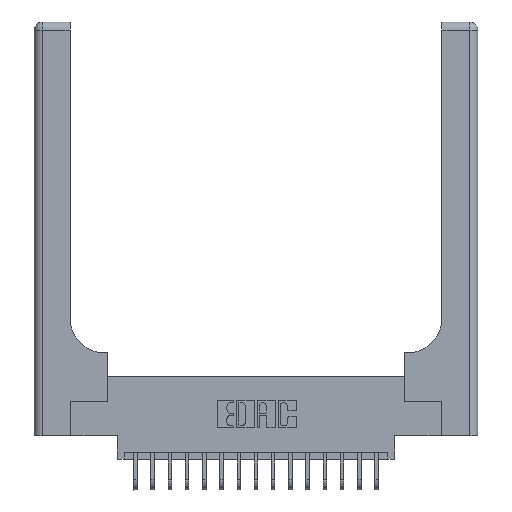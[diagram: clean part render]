
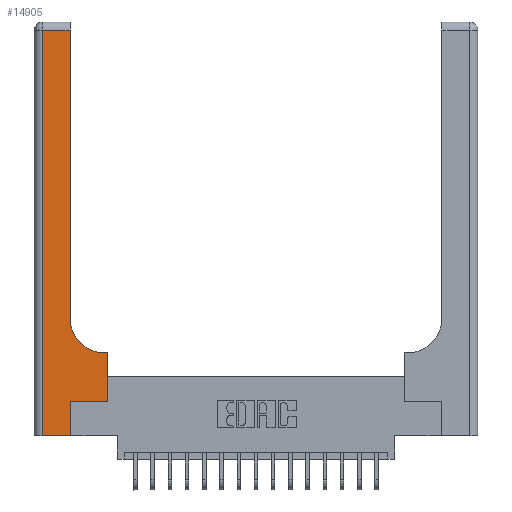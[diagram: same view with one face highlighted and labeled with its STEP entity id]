
A CAD part, top view. The second image highlights one B-rep face of the part: STEP entity #14905.
In plain terms, the highlighted planar face has unit normal (0, 0, 1).
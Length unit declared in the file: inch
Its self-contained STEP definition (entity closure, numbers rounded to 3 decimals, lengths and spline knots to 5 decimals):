
#407 = LINE ( 'NONE', #10503, #17776 ) ;
#1780 = VERTEX_POINT ( 'NONE', #20409 ) ;
#2011 = LINE ( 'NONE', #2367, #18367 ) ;
#2169 = EDGE_CURVE ( 'NONE', #14333, #17409, #12651, .T. ) ;
#2367 = CARTESIAN_POINT ( 'NONE',  ( 0.528, 0.25, 0.37 ) ) ;
#2661 = AXIS2_PLACEMENT_3D ( 'NONE', #9910, #19460, #16227 ) ;
#2768 = ORIENTED_EDGE ( 'NONE', *, *, #6752, .T. ) ;
#3006 = CIRCLE ( 'NONE', #2661, 0.25 ) ;
#3217 = VERTEX_POINT ( 'NONE', #18694 ) ;
#3454 = CARTESIAN_POINT ( 'NONE',  ( 0.265, 0., 0.37 ) ) ;
#3527 = ORIENTED_EDGE ( 'NONE', *, *, #14203, .T. ) ;
#3906 = ORIENTED_EDGE ( 'NONE', *, *, #14160, .T. ) ;
#4637 = EDGE_CURVE ( 'NONE', #3217, #15013, #407, .T. ) ;
#4768 = CARTESIAN_POINT ( 'NONE',  ( 0.26, 2.94, 0.37 ) ) ;
#5118 = CARTESIAN_POINT ( 'NONE',  ( 0.26, 0.6, 0.37 ) ) ;
#5528 = DIRECTION ( 'NONE',  ( 1., 0., 0. ) ) ;
#5822 = EDGE_CURVE ( 'NONE', #13208, #17805, #9298, .T. ) ;
#6103 = CARTESIAN_POINT ( 'NONE',  ( 0.06, 2.94, 0.37 ) ) ;
#6664 = FACE_OUTER_BOUND ( 'NONE', #16321, .T. ) ;
#6752 = EDGE_CURVE ( 'NONE', #17409, #18401, #16441, .T. ) ;
#7077 = CARTESIAN_POINT ( 'NONE',  ( 0.26, 0.85, 0.37 ) ) ;
#7537 = LINE ( 'NONE', #7980, #16976 ) ;
#7801 = DIRECTION ( 'NONE',  ( -1., 0., 0. ) ) ;
#7980 = CARTESIAN_POINT ( 'NONE',  ( 0., 0., 0.37 ) ) ;
#8175 = DIRECTION ( 'NONE',  ( 1., 0., 0. ) ) ;
#8461 = CARTESIAN_POINT ( 'NONE',  ( 0.528, 0.6, 0.37 ) ) ;
#8627 = EDGE_CURVE ( 'NONE', #11058, #3217, #8779, .T. ) ;
#8661 = EDGE_CURVE ( 'NONE', #1780, #11058, #7537, .T. ) ;
#8779 = LINE ( 'NONE', #14369, #16446 ) ;
#9016 = VECTOR ( 'NONE', #7801, 39.37008 ) ;
#9060 = ORIENTED_EDGE ( 'NONE', *, *, #4637, .T. ) ;
#9298 = LINE ( 'NONE', #5118, #17259 ) ;
#9910 = CARTESIAN_POINT ( 'NONE',  ( 0.51, 0.85, 0.37 ) ) ;
#10046 = AXIS2_PLACEMENT_3D ( 'NONE', #15260, #16838, #13586 ) ;
#10503 = CARTESIAN_POINT ( 'NONE',  ( 0.265, 0.25, 0.37 ) ) ;
#10622 = DIRECTION ( 'NONE',  ( 0., 1., 0. ) ) ;
#10773 = CARTESIAN_POINT ( 'NONE',  ( 0.528, 0.25, 0.37 ) ) ;
#10827 = CARTESIAN_POINT ( 'NONE',  ( 0.26, 3., 0.37 ) ) ;
#11058 = VERTEX_POINT ( 'NONE', #3454 ) ;
#11066 = DIRECTION ( 'NONE',  ( 0., 1., 0. ) ) ;
#11326 = EDGE_CURVE ( 'NONE', #15013, #13208, #2011, .T. ) ;
#11498 = CARTESIAN_POINT ( 'NONE',  ( 0.06, 3., 0.37 ) ) ;
#11913 = VECTOR ( 'NONE', #14733, 39.37008 ) ;
#12144 = VECTOR ( 'NONE', #10622, 39.37008 ) ;
#12651 = LINE ( 'NONE', #10827, #12144 ) ;
#13208 = VERTEX_POINT ( 'NONE', #8461 ) ;
#13443 = DIRECTION ( 'NONE',  ( 0., 1., 0. ) ) ;
#13586 = DIRECTION ( 'NONE',  ( -1., 0., 0. ) ) ;
#13652 = CARTESIAN_POINT ( 'NONE',  ( 0.51, 0.6, 0.37 ) ) ;
#13724 = ORIENTED_EDGE ( 'NONE', *, *, #2169, .T. ) ;
#13742 = ORIENTED_EDGE ( 'NONE', *, *, #5822, .T. ) ;
#14160 = EDGE_CURVE ( 'NONE', #17805, #14333, #3006, .T. ) ;
#14203 = EDGE_CURVE ( 'NONE', #18401, #1780, #14666, .T. ) ;
#14333 = VERTEX_POINT ( 'NONE', #7077 ) ;
#14369 = CARTESIAN_POINT ( 'NONE',  ( 0.265, 0., 0.37 ) ) ;
#14666 = LINE ( 'NONE', #11498, #11913 ) ;
#14710 = DIRECTION ( 'NONE',  ( -1., 0., 0. ) ) ;
#14733 = DIRECTION ( 'NONE',  ( 0., -1., 0. ) ) ;
#14905 = ADVANCED_FACE ( 'NONE', ( #6664 ), #18243, .F. ) ;
#15013 = VERTEX_POINT ( 'NONE', #10773 ) ;
#15260 = CARTESIAN_POINT ( 'NONE',  ( 0., 3., 0.37 ) ) ;
#15508 = ORIENTED_EDGE ( 'NONE', *, *, #8627, .T. ) ;
#15815 = ORIENTED_EDGE ( 'NONE', *, *, #11326, .T. ) ;
#15863 = CARTESIAN_POINT ( 'NONE',  ( 0., 2.94, 0.37 ) ) ;
#16227 = DIRECTION ( 'NONE',  ( 1., 0., 0. ) ) ;
#16321 = EDGE_LOOP ( 'NONE', ( #13724, #2768, #3527, #19326, #15508, #9060, #15815, #13742, #3906 ) ) ;
#16441 = LINE ( 'NONE', #15863, #9016 ) ;
#16446 = VECTOR ( 'NONE', #11066, 39.37008 ) ;
#16838 = DIRECTION ( 'NONE',  ( 0., 0., -1. ) ) ;
#16976 = VECTOR ( 'NONE', #8175, 39.37008 ) ;
#17259 = VECTOR ( 'NONE', #14710, 39.37008 ) ;
#17409 = VERTEX_POINT ( 'NONE', #4768 ) ;
#17776 = VECTOR ( 'NONE', #5528, 39.37008 ) ;
#17805 = VERTEX_POINT ( 'NONE', #13652 ) ;
#18243 = PLANE ( 'NONE',  #10046 ) ;
#18367 = VECTOR ( 'NONE', #13443, 39.37008 ) ;
#18401 = VERTEX_POINT ( 'NONE', #6103 ) ;
#18694 = CARTESIAN_POINT ( 'NONE',  ( 0.265, 0.25, 0.37 ) ) ;
#19326 = ORIENTED_EDGE ( 'NONE', *, *, #8661, .T. ) ;
#19460 = DIRECTION ( 'NONE',  ( 0., 0., -1. ) ) ;
#20409 = CARTESIAN_POINT ( 'NONE',  ( 0.06, 0., 0.37 ) ) ;
